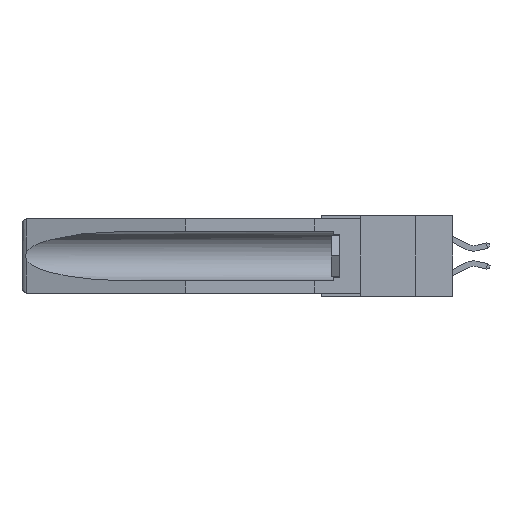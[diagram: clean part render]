
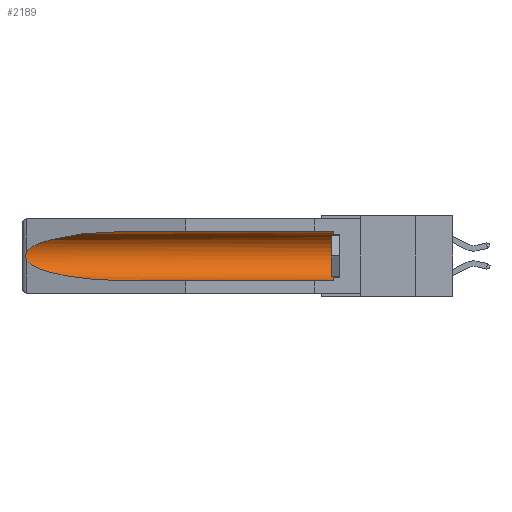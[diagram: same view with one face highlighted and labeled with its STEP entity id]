
A CAD part, left-side view. The second image highlights one B-rep face of the part: STEP entity #2189.
In plain terms, the highlighted cylindrical face has radius 2.857 mm (diameter 5.715 mm), a partial arc.
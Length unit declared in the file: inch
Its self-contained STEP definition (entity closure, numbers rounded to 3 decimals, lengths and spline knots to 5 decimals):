
#811 = CARTESIAN_POINT ( 'NONE',  ( 0.21114, 1.30732, -0.059 ) ) ;
#1186 = CARTESIAN_POINT ( 'NONE',  ( 0.26537, 1.52718, -0.14972 ) ) ;
#1316 = EDGE_CURVE ( 'NONE', #7339, #17034, #21423, .T. ) ;
#1549 = CARTESIAN_POINT ( 'NONE',  ( 0.25451, 1.48313, -0.09465 ) ) ;
#2183 = EDGE_CURVE ( 'NONE', #15878, #19248, #7354, .T. ) ;
#2189 = ADVANCED_FACE ( 'NONE', ( #17771 ), #14892, .F. ) ;
#2452 = ORIENTED_EDGE ( 'NONE', *, *, #5617, .T. ) ;
#3273 = CARTESIAN_POINT ( 'NONE',  ( 0.25451, 1.48313, -0.24835 ) ) ;
#3319 = ORIENTED_EDGE ( 'NONE', *, *, #21902, .T. ) ;
#4751 = VERTEX_POINT ( 'NONE', #25773 ) ;
#4991 = DIRECTION ( 'NONE',  ( 0., 1., 0. ) ) ;
#5453 = VERTEX_POINT ( 'NONE', #24209 ) ;
#5518 = ORIENTED_EDGE ( 'NONE', *, *, #18685, .T. ) ;
#5541 = CARTESIAN_POINT ( 'NONE',  ( 0.26597, 1.52961, -0.15275 ) ) ;
#5617 = EDGE_CURVE ( 'NONE', #5453, #15878, #14547, .T. ) ;
#6891 = CARTESIAN_POINT ( 'NONE',  ( 0.26537, 1.52718, -0.14972 ) ) ;
#7004 = CARTESIAN_POINT ( 'NONE',  ( 0.155, -0.30754, -0.059 ) ) ;
#7339 = VERTEX_POINT ( 'NONE', #13134 ) ;
#7354 = B_SPLINE_CURVE_WITH_KNOTS ( 'NONE', 3,
 ( #20240, #5541, #7558, #22229, #20072, #11740, #26249, #26430, #11821, #26339 ),
 .UNSPECIFIED., .F., .F.,
 ( 4, 2, 2, 2, 4 ),
 ( 0., 0.00029, 0.00058, 0.00087, 0.00117 ),
 .UNSPECIFIED. ) ;
#7558 = CARTESIAN_POINT ( 'NONE',  ( 0.26654, 1.53092, -0.15636 ) ) ;
#7929 = DIRECTION ( 'NONE',  ( 0., 1., 0. ) ) ;
#9208 = CARTESIAN_POINT ( 'NONE',  ( 0.26537, 1.52718, -0.19328 ) ) ;
#10826 = ORIENTED_EDGE ( 'NONE', *, *, #1316, .F. ) ;
#11183 = DIRECTION ( 'NONE',  ( 0., 1., 0. ) ) ;
#11740 = CARTESIAN_POINT ( 'NONE',  ( 0.2675, 1.53308, -0.17534 ) ) ;
#11821 = CARTESIAN_POINT ( 'NONE',  ( 0.26597, 1.5296, -0.19026 ) ) ;
#13054 = EDGE_CURVE ( 'NONE', #7339, #4751, #25071, .T. ) ;
#13134 = CARTESIAN_POINT ( 'NONE',  ( 0.155, 0.126, -0.284 ) ) ;
#13270 = CARTESIAN_POINT ( 'NONE',  ( 0.155, -0.30754, -0.1715 ) ) ;
#14547 =( BOUNDED_CURVE ( )  B_SPLINE_CURVE ( 3, ( #15328, #811, #1549, #1186 ),
 .UNSPECIFIED., .F., .F. ) 
 B_SPLINE_CURVE_WITH_KNOTS ( ( 4, 4 ),
 ( 4.71239, 6.08839 ),
 .UNSPECIFIED. ) 
 CURVE ( )  GEOMETRIC_REPRESENTATION_ITEM ( )  RATIONAL_B_SPLINE_CURVE ( ( 1., 0.848, 0.848, 1. ) ) 
 REPRESENTATION_ITEM ( '' )  );
#14651 = AXIS2_PLACEMENT_3D ( 'NONE', #13270, #4991, #18174 ) ;
#14892 = CYLINDRICAL_SURFACE ( 'NONE', #14651, 0.1125 ) ;
#14981 = ORIENTED_EDGE ( 'NONE', *, *, #2183, .T. ) ;
#15328 = CARTESIAN_POINT ( 'NONE',  ( 0.155, 1.07973, -0.059 ) ) ;
#15878 = VERTEX_POINT ( 'NONE', #6891 ) ;
#16186 = CARTESIAN_POINT ( 'NONE',  ( 0.155, -0.30754, -0.284 ) ) ;
#17034 = VERTEX_POINT ( 'NONE', #22451 ) ;
#17287 = VECTOR ( 'NONE', #11183, 39.37008 ) ;
#17771 = FACE_OUTER_BOUND ( 'NONE', #21909, .T. ) ;
#18174 = DIRECTION ( 'NONE',  ( 0., 0., 1. ) ) ;
#18685 = EDGE_CURVE ( 'NONE', #4751, #5453, #21139, .T. ) ;
#19239 = CARTESIAN_POINT ( 'NONE',  ( 0.26537, 1.52718, -0.19328 ) ) ;
#19248 = VERTEX_POINT ( 'NONE', #19239 ) ;
#19823 = CARTESIAN_POINT ( 'NONE',  ( 0.21114, 1.30732, -0.284 ) ) ;
#19996 = AXIS2_PLACEMENT_3D ( 'NONE', #20277, #20018, #26571 ) ;
#20018 = DIRECTION ( 'NONE',  ( 0., -1., 0. ) ) ;
#20072 = CARTESIAN_POINT ( 'NONE',  ( 0.2675, 1.53308, -0.16763 ) ) ;
#20160 =( BOUNDED_CURVE ( )  B_SPLINE_CURVE ( 3, ( #9208, #3273, #19823, #21898 ),
 .UNSPECIFIED., .F., .F. ) 
 B_SPLINE_CURVE_WITH_KNOTS ( ( 4, 4 ),
 ( 0.1948, 1.5708 ),
 .UNSPECIFIED. ) 
 CURVE ( )  GEOMETRIC_REPRESENTATION_ITEM ( )  RATIONAL_B_SPLINE_CURVE ( ( 1., 0.848, 0.848, 1. ) ) 
 REPRESENTATION_ITEM ( '' )  );
#20189 = ORIENTED_EDGE ( 'NONE', *, *, #13054, .T. ) ;
#20240 = CARTESIAN_POINT ( 'NONE',  ( 0.26537, 1.52718, -0.14972 ) ) ;
#20277 = CARTESIAN_POINT ( 'NONE',  ( 0.155, 0.126, -0.1715 ) ) ;
#21139 = LINE ( 'NONE', #7004, #17287 ) ;
#21423 = LINE ( 'NONE', #16186, #23682 ) ;
#21898 = CARTESIAN_POINT ( 'NONE',  ( 0.155, 1.07973, -0.284 ) ) ;
#21902 = EDGE_CURVE ( 'NONE', #19248, #17034, #20160, .T. ) ;
#21909 = EDGE_LOOP ( 'NONE', ( #2452, #14981, #3319, #10826, #20189, #5518 ) ) ;
#22229 = CARTESIAN_POINT ( 'NONE',  ( 0.2673, 1.5327, -0.16383 ) ) ;
#22451 = CARTESIAN_POINT ( 'NONE',  ( 0.155, 1.07973, -0.284 ) ) ;
#23682 = VECTOR ( 'NONE', #7929, 39.37008 ) ;
#24209 = CARTESIAN_POINT ( 'NONE',  ( 0.155, 1.07973, -0.059 ) ) ;
#25071 = CIRCLE ( 'NONE', #19996, 0.1125 ) ;
#25773 = CARTESIAN_POINT ( 'NONE',  ( 0.155, 0.126, -0.059 ) ) ;
#26249 = CARTESIAN_POINT ( 'NONE',  ( 0.2673, 1.53269, -0.17917 ) ) ;
#26339 = CARTESIAN_POINT ( 'NONE',  ( 0.26537, 1.52718, -0.19328 ) ) ;
#26430 = CARTESIAN_POINT ( 'NONE',  ( 0.26655, 1.53094, -0.18657 ) ) ;
#26571 = DIRECTION ( 'NONE',  ( 0., 0., 1. ) ) ;
